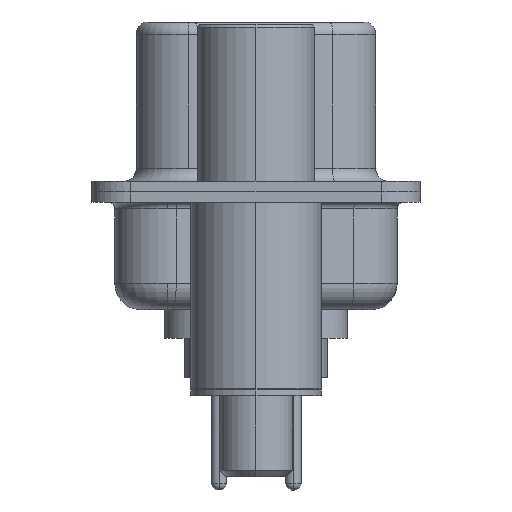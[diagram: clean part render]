
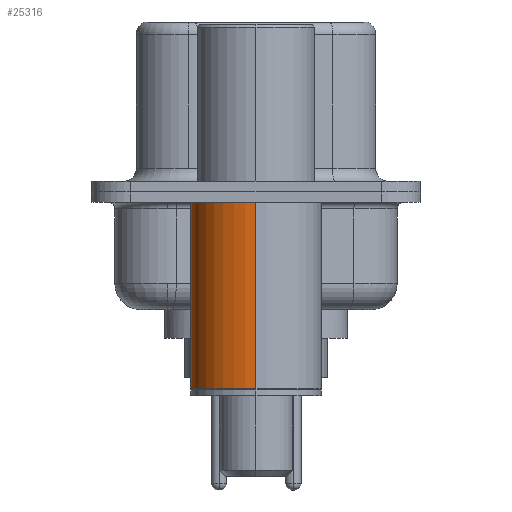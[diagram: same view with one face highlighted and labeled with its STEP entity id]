
A CAD part, left-side view. The second image highlights one B-rep face of the part: STEP entity #25316.
In plain terms, the highlighted cylindrical face has radius 2.5 mm (diameter 5 mm), a partial arc.
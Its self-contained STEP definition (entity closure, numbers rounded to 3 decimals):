
#3325 = EDGE_CURVE ( 'NONE', #23371, #10997, #20306, .T. ) ;
#3395 = ORIENTED_EDGE ( 'NONE', *, *, #3325, .T. ) ;
#4213 = AXIS2_PLACEMENT_3D ( 'NONE', #6605, #20279, #8561 ) ;
#6605 = CARTESIAN_POINT ( 'NONE',  ( 0., 0., -0.4 ) ) ;
#7805 = EDGE_LOOP ( 'NONE', ( #3395, #18169, #23611, #24643 ) ) ;
#7913 = CARTESIAN_POINT ( 'NONE',  ( 2.5, 0., -7.525 ) ) ;
#8102 = CYLINDRICAL_SURFACE ( 'NONE', #24042, 2.5 ) ;
#8550 = VERTEX_POINT ( 'NONE', #21688 ) ;
#8561 = DIRECTION ( 'NONE',  ( 1., 0., 0. ) ) ;
#10505 = DIRECTION ( 'NONE',  ( 0., 0., 1. ) ) ;
#10997 = VERTEX_POINT ( 'NONE', #20704 ) ;
#11084 = DIRECTION ( 'NONE',  ( 0., 0., 1. ) ) ;
#11667 = VECTOR ( 'NONE', #14297, 1000. ) ;
#12338 = CARTESIAN_POINT ( 'NONE',  ( -2.5, 0., 0.581 ) ) ;
#13084 = AXIS2_PLACEMENT_3D ( 'NONE', #22821, #11084, #24802 ) ;
#13573 = CIRCLE ( 'NONE', #4213, 2.5 ) ;
#13911 = FACE_OUTER_BOUND ( 'NONE', #7805, .T. ) ;
#14297 = DIRECTION ( 'NONE',  ( 0., 0., 1. ) ) ;
#15711 = DIRECTION ( 'NONE',  ( 0., 0., 1. ) ) ;
#16707 = VECTOR ( 'NONE', #10505, 1000. ) ;
#16894 = EDGE_CURVE ( 'NONE', #8550, #16952, #13573, .T. ) ;
#16952 = VERTEX_POINT ( 'NONE', #20458 ) ;
#17611 = DIRECTION ( 'NONE',  ( 1., 0., 0. ) ) ;
#17686 = CARTESIAN_POINT ( 'NONE',  ( 0., 0., 0.581 ) ) ;
#18169 = ORIENTED_EDGE ( 'NONE', *, *, #18887, .T. ) ;
#18887 = EDGE_CURVE ( 'NONE', #10997, #16952, #21454, .T. ) ;
#20279 = DIRECTION ( 'NONE',  ( 0., 0., 1. ) ) ;
#20306 = CIRCLE ( 'NONE', #13084, 2.5 ) ;
#20458 = CARTESIAN_POINT ( 'NONE',  ( -2.5, 0., -0.4 ) ) ;
#20704 = CARTESIAN_POINT ( 'NONE',  ( -2.5, 0., -7.525 ) ) ;
#21454 = LINE ( 'NONE', #12338, #11667 ) ;
#21688 = CARTESIAN_POINT ( 'NONE',  ( 2.5, 0., -0.4 ) ) ;
#21910 = LINE ( 'NONE', #22250, #16707 ) ;
#22250 = CARTESIAN_POINT ( 'NONE',  ( 2.5, 0., 0.581 ) ) ;
#22821 = CARTESIAN_POINT ( 'NONE',  ( 0., 0., -7.525 ) ) ;
#23371 = VERTEX_POINT ( 'NONE', #7913 ) ;
#23611 = ORIENTED_EDGE ( 'NONE', *, *, #16894, .F. ) ;
#24042 = AXIS2_PLACEMENT_3D ( 'NONE', #17686, #15711, #17611 ) ;
#24643 = ORIENTED_EDGE ( 'NONE', *, *, #24967, .F. ) ;
#24802 = DIRECTION ( 'NONE',  ( 1., 0., 0. ) ) ;
#24967 = EDGE_CURVE ( 'NONE', #23371, #8550, #21910, .T. ) ;
#25316 = ADVANCED_FACE ( 'NONE', ( #13911 ), #8102, .T. ) ;
